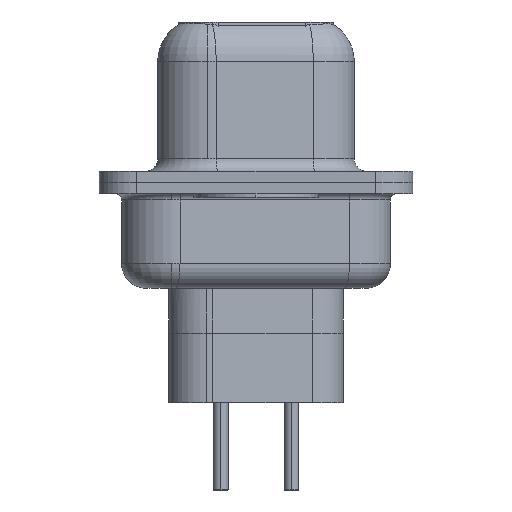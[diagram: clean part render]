
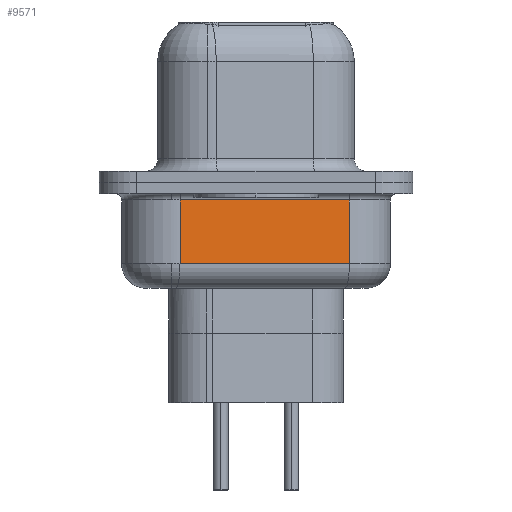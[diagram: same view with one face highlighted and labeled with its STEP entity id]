
A CAD part, left-side view. The second image highlights one B-rep face of the part: STEP entity #9571.
In plain terms, the highlighted planar face has unit normal (-0.985, -0.174, 0).
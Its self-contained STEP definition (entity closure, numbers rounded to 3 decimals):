
#2101 = VECTOR ( 'NONE', #15407, 1000. ) ;
#2815 = CARTESIAN_POINT ( 'NONE',  ( 4.074, -3.747, -4.25 ) ) ;
#2831 = VERTEX_POINT ( 'NONE', #7789 ) ;
#3475 = VERTEX_POINT ( 'NONE', #15451 ) ;
#3973 = CARTESIAN_POINT ( 'NONE',  ( 2.875, 3.053, -4.25 ) ) ;
#4162 = EDGE_CURVE ( 'NONE', #17435, #3475, #18429, .T. ) ;
#4390 = LINE ( 'NONE', #2815, #2101 ) ;
#4884 = CARTESIAN_POINT ( 'NONE',  ( 4.074, -3.747, -0.7 ) ) ;
#5339 = DIRECTION ( 'NONE',  ( 0.985, 0.174, 0. ) ) ;
#6235 = ORIENTED_EDGE ( 'NONE', *, *, #7113, .T. ) ;
#7113 = EDGE_CURVE ( 'NONE', #12125, #3475, #14827, .T. ) ;
#7282 = CARTESIAN_POINT ( 'NONE',  ( 2.875, 3.053, -3.25 ) ) ;
#7789 = CARTESIAN_POINT ( 'NONE',  ( 4.074, -3.747, -3.25 ) ) ;
#8941 = DIRECTION ( 'NONE',  ( 0., 0., 1. ) ) ;
#9571 = ADVANCED_FACE ( 'NONE', ( #15279 ), #14967, .F. ) ;
#10070 = DIRECTION ( 'NONE',  ( -0.174, 0.985, 0. ) ) ;
#10186 = VECTOR ( 'NONE', #17743, 1000. ) ;
#11670 = CARTESIAN_POINT ( 'NONE',  ( 2.875, 3.053, -0.7 ) ) ;
#11761 = AXIS2_PLACEMENT_3D ( 'NONE', #3973, #5339, #16656 ) ;
#12125 = VERTEX_POINT ( 'NONE', #4884 ) ;
#13191 = LINE ( 'NONE', #19429, #10186 ) ;
#13304 = EDGE_CURVE ( 'NONE', #2831, #12125, #4390, .T. ) ;
#14104 = EDGE_CURVE ( 'NONE', #17435, #2831, #13191, .T. ) ;
#14788 = ORIENTED_EDGE ( 'NONE', *, *, #13304, .T. ) ;
#14827 = LINE ( 'NONE', #11670, #19658 ) ;
#14967 = PLANE ( 'NONE',  #11761 ) ;
#15279 = FACE_OUTER_BOUND ( 'NONE', #18270, .T. ) ;
#15407 = DIRECTION ( 'NONE',  ( 0., 0., 1. ) ) ;
#15451 = CARTESIAN_POINT ( 'NONE',  ( 2.875, 3.053, -0.7 ) ) ;
#16422 = ORIENTED_EDGE ( 'NONE', *, *, #4162, .F. ) ;
#16513 = VECTOR ( 'NONE', #8941, 1000. ) ;
#16656 = DIRECTION ( 'NONE',  ( -0.174, 0.985, 0. ) ) ;
#17165 = CARTESIAN_POINT ( 'NONE',  ( 2.875, 3.053, -4.25 ) ) ;
#17412 = ORIENTED_EDGE ( 'NONE', *, *, #14104, .T. ) ;
#17435 = VERTEX_POINT ( 'NONE', #7282 ) ;
#17743 = DIRECTION ( 'NONE',  ( 0.174, -0.985, 0. ) ) ;
#18270 = EDGE_LOOP ( 'NONE', ( #16422, #17412, #14788, #6235 ) ) ;
#18429 = LINE ( 'NONE', #17165, #16513 ) ;
#19429 = CARTESIAN_POINT ( 'NONE',  ( 2.875, 3.053, -3.25 ) ) ;
#19658 = VECTOR ( 'NONE', #10070, 1000. ) ;
